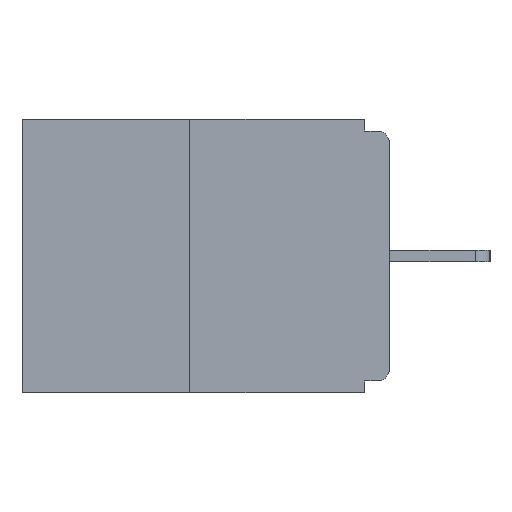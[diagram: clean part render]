
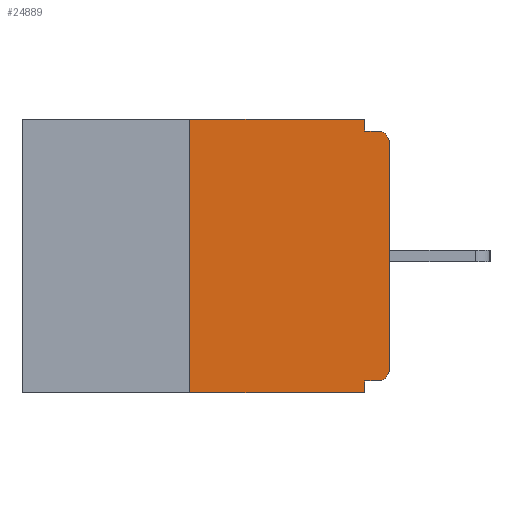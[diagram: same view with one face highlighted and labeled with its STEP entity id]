
A CAD part, left-side view. The second image highlights one B-rep face of the part: STEP entity #24889.
In plain terms, the highlighted planar face has unit normal (-1, 0, 0).
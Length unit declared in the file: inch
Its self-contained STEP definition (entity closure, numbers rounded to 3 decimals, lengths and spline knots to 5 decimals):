
#745 = CARTESIAN_POINT ( 'NONE',  ( 0., 0.46, -0.343 ) ) ;
#811 = DIRECTION ( 'NONE',  ( 0., -1., 0. ) ) ;
#1062 = VECTOR ( 'NONE', #13531, 39.37008 ) ;
#1486 = AXIS2_PLACEMENT_3D ( 'NONE', #6335, #16301, #16173 ) ;
#1734 = LINE ( 'NONE', #9729, #8516 ) ;
#1929 = EDGE_CURVE ( 'NONE', #18308, #12472, #12677, .T. ) ;
#2263 = CARTESIAN_POINT ( 'NONE',  ( 0., 0.25, 0. ) ) ;
#2416 = VERTEX_POINT ( 'NONE', #18890 ) ;
#2786 = EDGE_CURVE ( 'NONE', #16761, #4407, #13000, .T. ) ;
#2930 = CARTESIAN_POINT ( 'NONE',  ( 0., 0.031, -0.328 ) ) ;
#3123 = VERTEX_POINT ( 'NONE', #10106 ) ;
#3304 = CARTESIAN_POINT ( 'NONE',  ( 0., 0.46, 0. ) ) ;
#3785 = CARTESIAN_POINT ( 'NONE',  ( 0., 0.031, 0. ) ) ;
#4020 = CARTESIAN_POINT ( 'NONE',  ( 0., 0.031, 0. ) ) ;
#4033 = DIRECTION ( 'NONE',  ( 0., 1., 0. ) ) ;
#4407 = VERTEX_POINT ( 'NONE', #21454 ) ;
#4446 = EDGE_CURVE ( 'NONE', #2416, #11720, #20354, .T. ) ;
#4929 = EDGE_CURVE ( 'NONE', #2416, #3123, #17376, .T. ) ;
#5377 = DIRECTION ( 'NONE',  ( 0., 0., -1. ) ) ;
#5644 = EDGE_CURVE ( 'NONE', #8911, #16775, #9473, .T. ) ;
#5765 = VECTOR ( 'NONE', #4033, 39.37008 ) ;
#5877 = CARTESIAN_POINT ( 'NONE',  ( 0., 0.25, 0. ) ) ;
#6335 = CARTESIAN_POINT ( 'NONE',  ( 0., 0.015, -0.313 ) ) ;
#6344 = EDGE_LOOP ( 'NONE', ( #21015, #15562, #20107, #6766, #15936, #16763, #19611, #23038, #8554, #17572 ) ) ;
#6766 = ORIENTED_EDGE ( 'NONE', *, *, #25833, .F. ) ;
#7017 = DIRECTION ( 'NONE',  ( 0., -1., 0. ) ) ;
#7150 = CARTESIAN_POINT ( 'NONE',  ( 0., 0.46, 0. ) ) ;
#7457 = CARTESIAN_POINT ( 'NONE',  ( 0., 0., -0.03 ) ) ;
#8516 = VECTOR ( 'NONE', #23951, 39.37008 ) ;
#8554 = ORIENTED_EDGE ( 'NONE', *, *, #2786, .F. ) ;
#8911 = VERTEX_POINT ( 'NONE', #5877 ) ;
#9473 = LINE ( 'NONE', #3304, #1062 ) ;
#9729 = CARTESIAN_POINT ( 'NONE',  ( 0., 0.031, -0.343 ) ) ;
#10106 = CARTESIAN_POINT ( 'NONE',  ( 0., 0., -0.313 ) ) ;
#10280 = DIRECTION ( 'NONE',  ( 0., 0., 1. ) ) ;
#11181 = DIRECTION ( 'NONE',  ( -1., 0., 0. ) ) ;
#11241 = AXIS2_PLACEMENT_3D ( 'NONE', #24877, #11181, #5377 ) ;
#11377 = DIRECTION ( 'NONE',  ( 0., 0., -1. ) ) ;
#11508 = FACE_OUTER_BOUND ( 'NONE', #6344, .T. ) ;
#11720 = VERTEX_POINT ( 'NONE', #2930 ) ;
#12168 = CARTESIAN_POINT ( 'NONE',  ( 0., 0.031, -0.015 ) ) ;
#12398 = EDGE_CURVE ( 'NONE', #24517, #4407, #22898, .T. ) ;
#12472 = VERTEX_POINT ( 'NONE', #19620 ) ;
#12538 = VECTOR ( 'NONE', #20969, 39.37008 ) ;
#12677 = LINE ( 'NONE', #745, #25084 ) ;
#13000 = LINE ( 'NONE', #18720, #14810 ) ;
#13531 = DIRECTION ( 'NONE',  ( 0., -1., 0. ) ) ;
#14018 = DIRECTION ( 'NONE',  ( 0., 0., -1. ) ) ;
#14810 = VECTOR ( 'NONE', #811, 39.37008 ) ;
#15515 = VECTOR ( 'NONE', #14018, 39.37008 ) ;
#15561 = EDGE_CURVE ( 'NONE', #18308, #8911, #22799, .T. ) ;
#15562 = ORIENTED_EDGE ( 'NONE', *, *, #15561, .F. ) ;
#15936 = ORIENTED_EDGE ( 'NONE', *, *, #4446, .F. ) ;
#15957 = LINE ( 'NONE', #3785, #15515 ) ;
#16173 = DIRECTION ( 'NONE',  ( 0., 0., -1. ) ) ;
#16301 = DIRECTION ( 'NONE',  ( -1., 0., 0. ) ) ;
#16663 = LINE ( 'NONE', #22792, #12538 ) ;
#16761 = VERTEX_POINT ( 'NONE', #12168 ) ;
#16763 = ORIENTED_EDGE ( 'NONE', *, *, #4929, .T. ) ;
#16775 = VERTEX_POINT ( 'NONE', #4020 ) ;
#17238 = PLANE ( 'NONE',  #19745 ) ;
#17376 = CIRCLE ( 'NONE', #1486, 0.015 ) ;
#17572 = ORIENTED_EDGE ( 'NONE', *, *, #20670, .F. ) ;
#17619 = DIRECTION ( 'NONE',  ( 1., 0., 0. ) ) ;
#18308 = VERTEX_POINT ( 'NONE', #23503 ) ;
#18720 = CARTESIAN_POINT ( 'NONE',  ( 0., 0., -0.015 ) ) ;
#18890 = CARTESIAN_POINT ( 'NONE',  ( 0., 0.015, -0.328 ) ) ;
#19203 = VECTOR ( 'NONE', #10280, 39.37008 ) ;
#19611 = ORIENTED_EDGE ( 'NONE', *, *, #19863, .T. ) ;
#19620 = CARTESIAN_POINT ( 'NONE',  ( 0., 0.031, -0.343 ) ) ;
#19745 = AXIS2_PLACEMENT_3D ( 'NONE', #7150, #17619, #11377 ) ;
#19863 = EDGE_CURVE ( 'NONE', #3123, #24517, #16663, .T. ) ;
#19977 = CARTESIAN_POINT ( 'NONE',  ( 0., 0., -0.328 ) ) ;
#20107 = ORIENTED_EDGE ( 'NONE', *, *, #1929, .T. ) ;
#20354 = LINE ( 'NONE', #19977, #5765 ) ;
#20670 = EDGE_CURVE ( 'NONE', #16775, #16761, #15957, .T. ) ;
#20969 = DIRECTION ( 'NONE',  ( 0., 0., 1. ) ) ;
#21015 = ORIENTED_EDGE ( 'NONE', *, *, #5644, .F. ) ;
#21454 = CARTESIAN_POINT ( 'NONE',  ( 0., 0.015, -0.015 ) ) ;
#22792 = CARTESIAN_POINT ( 'NONE',  ( 0., 0., 0. ) ) ;
#22799 = LINE ( 'NONE', #2263, #19203 ) ;
#22898 = CIRCLE ( 'NONE', #11241, 0.015 ) ;
#23038 = ORIENTED_EDGE ( 'NONE', *, *, #12398, .T. ) ;
#23503 = CARTESIAN_POINT ( 'NONE',  ( 0., 0.25, -0.343 ) ) ;
#23951 = DIRECTION ( 'NONE',  ( 0., 0., -1. ) ) ;
#24517 = VERTEX_POINT ( 'NONE', #7457 ) ;
#24877 = CARTESIAN_POINT ( 'NONE',  ( 0., 0.015, -0.03 ) ) ;
#24889 = ADVANCED_FACE ( 'NONE', ( #11508 ), #17238, .F. ) ;
#25084 = VECTOR ( 'NONE', #7017, 39.37008 ) ;
#25833 = EDGE_CURVE ( 'NONE', #11720, #12472, #1734, .T. ) ;
